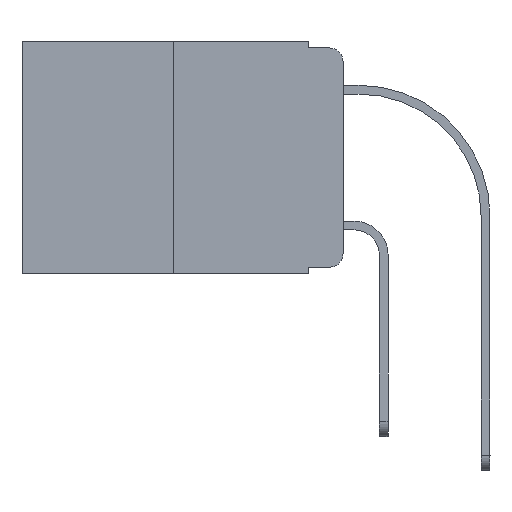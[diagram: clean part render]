
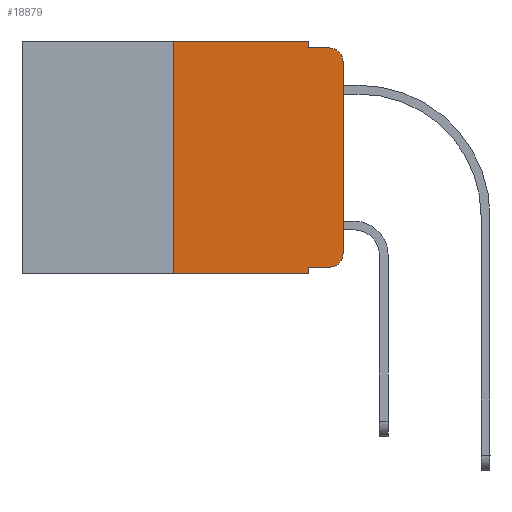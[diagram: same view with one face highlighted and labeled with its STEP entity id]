
A CAD part, left-side view. The second image highlights one B-rep face of the part: STEP entity #18879.
In plain terms, the highlighted planar face has unit normal (-1, 0, 0).
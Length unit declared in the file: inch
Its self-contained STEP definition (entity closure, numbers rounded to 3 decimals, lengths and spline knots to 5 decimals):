
#277 = DIRECTION ( 'NONE',  ( 0., 0., -1. ) ) ;
#396 = PLANE ( 'NONE',  #3744 ) ;
#670 = ORIENTED_EDGE ( 'NONE', *, *, #4281, .F. ) ;
#722 = DIRECTION ( 'NONE',  ( 1., 0., 0. ) ) ;
#820 = FACE_OUTER_BOUND ( 'NONE', #8538, .T. ) ;
#1037 = DIRECTION ( 'NONE',  ( 0., -1., 0. ) ) ;
#1419 = LINE ( 'NONE', #12997, #21323 ) ;
#1751 = LINE ( 'NONE', #13120, #5749 ) ;
#1787 = EDGE_CURVE ( 'NONE', #17244, #16553, #18415, .T. ) ;
#1799 = VERTEX_POINT ( 'NONE', #17236 ) ;
#1844 = ORIENTED_EDGE ( 'NONE', *, *, #4240, .T. ) ;
#1974 = VERTEX_POINT ( 'NONE', #19307 ) ;
#2794 = ORIENTED_EDGE ( 'NONE', *, *, #21483, .F. ) ;
#2884 = VERTEX_POINT ( 'NONE', #18933 ) ;
#3483 = VECTOR ( 'NONE', #1037, 39.37008 ) ;
#3744 = AXIS2_PLACEMENT_3D ( 'NONE', #18899, #722, #10786 ) ;
#4240 = EDGE_CURVE ( 'NONE', #15080, #11478, #16471, .T. ) ;
#4281 = EDGE_CURVE ( 'NONE', #4656, #1799, #1419, .T. ) ;
#4301 = CARTESIAN_POINT ( 'NONE',  ( 0., 0.473, 0. ) ) ;
#4354 = LINE ( 'NONE', #20774, #19845 ) ;
#4656 = VERTEX_POINT ( 'NONE', #12316 ) ;
#4768 = EDGE_CURVE ( 'NONE', #1974, #2884, #9896, .T. ) ;
#4898 = EDGE_CURVE ( 'NONE', #11478, #17244, #10522, .T. ) ;
#5622 = EDGE_CURVE ( 'NONE', #1799, #16553, #12991, .T. ) ;
#5749 = VECTOR ( 'NONE', #11479, 39.37008 ) ;
#5830 = ORIENTED_EDGE ( 'NONE', *, *, #5622, .F. ) ;
#6001 = DIRECTION ( 'NONE',  ( -1., 0., 0. ) ) ;
#6152 = VECTOR ( 'NONE', #6308, 39.37008 ) ;
#6308 = DIRECTION ( 'NONE',  ( 0., -1., 0. ) ) ;
#6322 = DIRECTION ( 'NONE',  ( 0., -1., 0. ) ) ;
#6739 = CARTESIAN_POINT ( 'NONE',  ( 0., 0.051, -0.01 ) ) ;
#7580 = ORIENTED_EDGE ( 'NONE', *, *, #7624, .F. ) ;
#7624 = EDGE_CURVE ( 'NONE', #8246, #4656, #15803, .T. ) ;
#7833 = CARTESIAN_POINT ( 'NONE',  ( 0., 0.473, -0.343 ) ) ;
#8246 = VERTEX_POINT ( 'NONE', #13019 ) ;
#8521 = EDGE_CURVE ( 'NONE', #19273, #15080, #19443, .T. ) ;
#8538 = EDGE_LOOP ( 'NONE', ( #9304, #14088, #5830, #670, #7580, #2794, #11763, #19665, #11773, #1844 ) ) ;
#9304 = ORIENTED_EDGE ( 'NONE', *, *, #4898, .T. ) ;
#9896 = LINE ( 'NONE', #7833, #6152 ) ;
#10522 = LINE ( 'NONE', #14030, #12458 ) ;
#10647 = CARTESIAN_POINT ( 'NONE',  ( 0., 0.02, -0.03 ) ) ;
#10786 = DIRECTION ( 'NONE',  ( 0., 0., -1. ) ) ;
#11120 = CARTESIAN_POINT ( 'NONE',  ( 0., 0.051, -0.333 ) ) ;
#11478 = VERTEX_POINT ( 'NONE', #11912 ) ;
#11479 = DIRECTION ( 'NONE',  ( 0., 0., 1. ) ) ;
#11599 = EDGE_CURVE ( 'NONE', #19273, #2884, #4354, .T. ) ;
#11763 = ORIENTED_EDGE ( 'NONE', *, *, #4768, .T. ) ;
#11773 = ORIENTED_EDGE ( 'NONE', *, *, #8521, .T. ) ;
#11912 = CARTESIAN_POINT ( 'NONE',  ( 0., 0., -0.313 ) ) ;
#12316 = CARTESIAN_POINT ( 'NONE',  ( 0., 0.051, 0. ) ) ;
#12458 = VECTOR ( 'NONE', #18863, 39.37008 ) ;
#12669 = DIRECTION ( 'NONE',  ( 0., 0., -1. ) ) ;
#12785 = VECTOR ( 'NONE', #17494, 39.37008 ) ;
#12991 = LINE ( 'NONE', #6739, #21597 ) ;
#12997 = CARTESIAN_POINT ( 'NONE',  ( 0., 0.051, 0. ) ) ;
#13019 = CARTESIAN_POINT ( 'NONE',  ( 0., 0.25, 0. ) ) ;
#13120 = CARTESIAN_POINT ( 'NONE',  ( 0., 0.25, 0. ) ) ;
#13951 = DIRECTION ( 'NONE',  ( -1., 0., 0. ) ) ;
#14030 = CARTESIAN_POINT ( 'NONE',  ( 0., 0., 0. ) ) ;
#14088 = ORIENTED_EDGE ( 'NONE', *, *, #1787, .T. ) ;
#15080 = VERTEX_POINT ( 'NONE', #19162 ) ;
#15757 = DIRECTION ( 'NONE',  ( 0., 0., -1. ) ) ;
#15803 = LINE ( 'NONE', #4301, #3483 ) ;
#16471 = CIRCLE ( 'NONE', #17524, 0.02 ) ;
#16553 = VERTEX_POINT ( 'NONE', #18265 ) ;
#17154 = CARTESIAN_POINT ( 'NONE',  ( 0., 0., -0.03 ) ) ;
#17236 = CARTESIAN_POINT ( 'NONE',  ( 0., 0.051, -0.01 ) ) ;
#17244 = VERTEX_POINT ( 'NONE', #17154 ) ;
#17494 = DIRECTION ( 'NONE',  ( 0., -1., 0. ) ) ;
#17524 = AXIS2_PLACEMENT_3D ( 'NONE', #21002, #6001, #12669 ) ;
#18265 = CARTESIAN_POINT ( 'NONE',  ( 0., 0.02, -0.01 ) ) ;
#18415 = CIRCLE ( 'NONE', #19460, 0.02 ) ;
#18863 = DIRECTION ( 'NONE',  ( 0., 0., 1. ) ) ;
#18879 = ADVANCED_FACE ( 'NONE', ( #820 ), #396, .F. ) ;
#18899 = CARTESIAN_POINT ( 'NONE',  ( 0., 0.473, 0. ) ) ;
#18933 = CARTESIAN_POINT ( 'NONE',  ( 0., 0.051, -0.343 ) ) ;
#19162 = CARTESIAN_POINT ( 'NONE',  ( 0., 0.02, -0.333 ) ) ;
#19273 = VERTEX_POINT ( 'NONE', #20060 ) ;
#19307 = CARTESIAN_POINT ( 'NONE',  ( 0., 0.25, -0.343 ) ) ;
#19443 = LINE ( 'NONE', #11120, #12785 ) ;
#19460 = AXIS2_PLACEMENT_3D ( 'NONE', #10647, #13951, #277 ) ;
#19665 = ORIENTED_EDGE ( 'NONE', *, *, #11599, .F. ) ;
#19681 = DIRECTION ( 'NONE',  ( 0., 0., -1. ) ) ;
#19845 = VECTOR ( 'NONE', #15757, 39.37008 ) ;
#20060 = CARTESIAN_POINT ( 'NONE',  ( 0., 0.051, -0.333 ) ) ;
#20774 = CARTESIAN_POINT ( 'NONE',  ( 0., 0.051, 0. ) ) ;
#21002 = CARTESIAN_POINT ( 'NONE',  ( 0., 0.02, -0.313 ) ) ;
#21323 = VECTOR ( 'NONE', #19681, 39.37008 ) ;
#21483 = EDGE_CURVE ( 'NONE', #1974, #8246, #1751, .T. ) ;
#21597 = VECTOR ( 'NONE', #6322, 39.37008 ) ;
